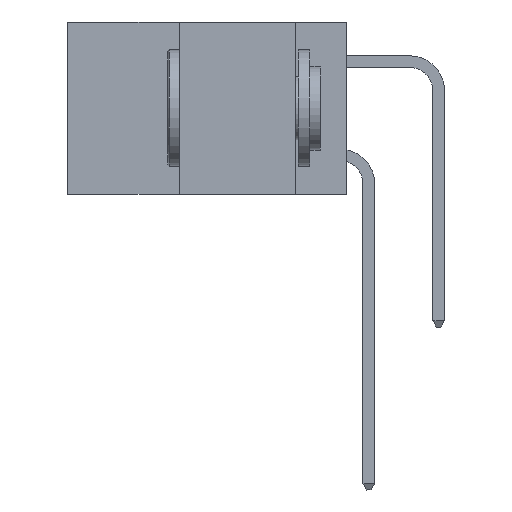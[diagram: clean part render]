
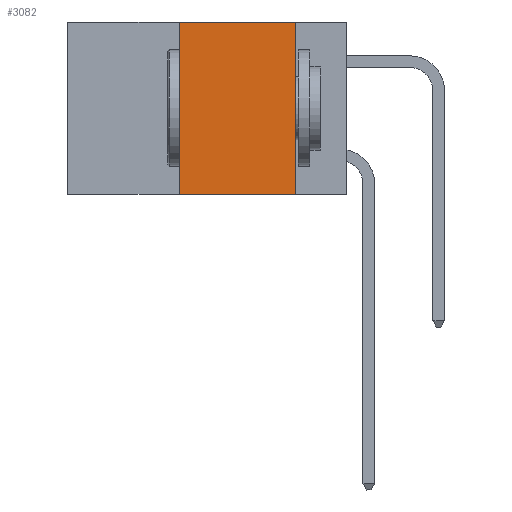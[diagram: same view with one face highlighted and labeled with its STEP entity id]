
A CAD part, left-side view. The second image highlights one B-rep face of the part: STEP entity #3082.
In plain terms, the highlighted planar face has unit normal (-1, 0, 0).
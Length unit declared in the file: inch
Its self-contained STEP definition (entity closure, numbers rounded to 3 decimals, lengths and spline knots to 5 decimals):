
#131 = AXIS2_PLACEMENT_3D ( 'NONE', #3730, #12913, #5605 ) ;
#1094 = DIRECTION ( 'NONE',  ( 0., -1., 0. ) ) ;
#1603 = PLANE ( 'NONE',  #131 ) ;
#1998 = FACE_OUTER_BOUND ( 'NONE', #4590, .T. ) ;
#2330 = VECTOR ( 'NONE', #11540, 39.37008 ) ;
#2653 = DIRECTION ( 'NONE',  ( 0., 0., -1. ) ) ;
#3082 = ADVANCED_FACE ( 'NONE', ( #1998 ), #1603, .F. ) ;
#3148 = EDGE_CURVE ( 'NONE', #8468, #10117, #8989, .T. ) ;
#3730 = CARTESIAN_POINT ( 'NONE',  ( 0., 0.6, 0. ) ) ;
#4437 = LINE ( 'NONE', #10878, #11507 ) ;
#4451 = CARTESIAN_POINT ( 'NONE',  ( 0., 0.11, 0. ) ) ;
#4590 = EDGE_LOOP ( 'NONE', ( #10039, #5751, #9449, #5336 ) ) ;
#5336 = ORIENTED_EDGE ( 'NONE', *, *, #7051, .T. ) ;
#5605 = DIRECTION ( 'NONE',  ( 0., 0., -1. ) ) ;
#5664 = CARTESIAN_POINT ( 'NONE',  ( 0., 0.11, 0. ) ) ;
#5751 = ORIENTED_EDGE ( 'NONE', *, *, #5861, .F. ) ;
#5861 = EDGE_CURVE ( 'NONE', #12023, #8468, #4437, .T. ) ;
#6078 = CARTESIAN_POINT ( 'NONE',  ( 0., 0.36, 0. ) ) ;
#6109 = VECTOR ( 'NONE', #2653, 39.37008 ) ;
#6341 = CARTESIAN_POINT ( 'NONE',  ( 0., 0.36, 0. ) ) ;
#6984 = EDGE_CURVE ( 'NONE', #9153, #12023, #10192, .T. ) ;
#7051 = EDGE_CURVE ( 'NONE', #9153, #10117, #9028, .T. ) ;
#7198 = CARTESIAN_POINT ( 'NONE',  ( 0., 0.6, -0.37 ) ) ;
#7277 = CARTESIAN_POINT ( 'NONE',  ( 0., 0.36, -0.37 ) ) ;
#8468 = VERTEX_POINT ( 'NONE', #4451 ) ;
#8989 = LINE ( 'NONE', #5664, #6109 ) ;
#9028 = LINE ( 'NONE', #7198, #12296 ) ;
#9153 = VERTEX_POINT ( 'NONE', #7277 ) ;
#9449 = ORIENTED_EDGE ( 'NONE', *, *, #6984, .F. ) ;
#10039 = ORIENTED_EDGE ( 'NONE', *, *, #3148, .F. ) ;
#10117 = VERTEX_POINT ( 'NONE', #10314 ) ;
#10192 = LINE ( 'NONE', #6341, #2330 ) ;
#10314 = CARTESIAN_POINT ( 'NONE',  ( 0., 0.11, -0.37 ) ) ;
#10878 = CARTESIAN_POINT ( 'NONE',  ( 0., 0.6, 0. ) ) ;
#11507 = VECTOR ( 'NONE', #12985, 39.37008 ) ;
#11540 = DIRECTION ( 'NONE',  ( 0., 0., 1. ) ) ;
#12023 = VERTEX_POINT ( 'NONE', #6078 ) ;
#12296 = VECTOR ( 'NONE', #1094, 39.37008 ) ;
#12913 = DIRECTION ( 'NONE',  ( 1., 0., 0. ) ) ;
#12985 = DIRECTION ( 'NONE',  ( 0., -1., 0. ) ) ;
